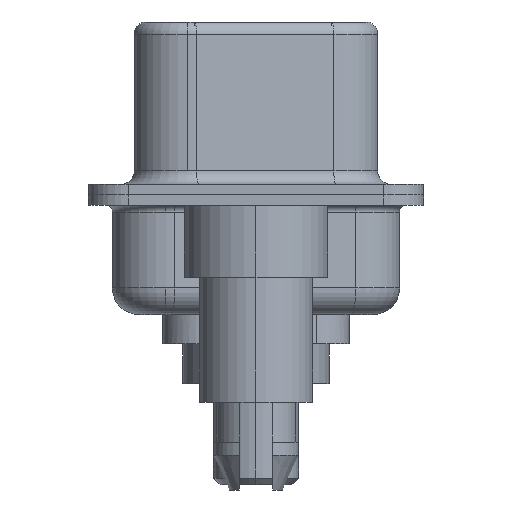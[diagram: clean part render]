
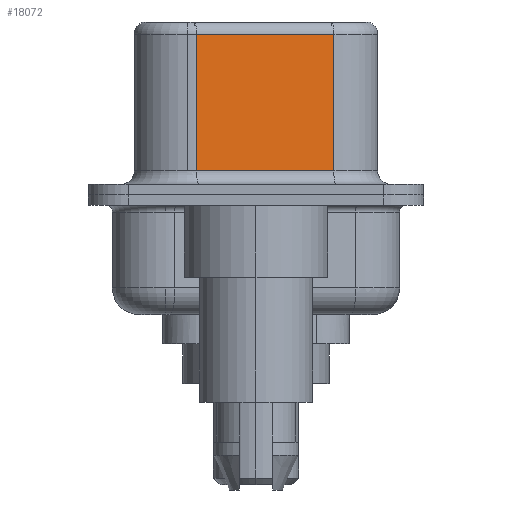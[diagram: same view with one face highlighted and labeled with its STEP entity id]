
A CAD part, left-side view. The second image highlights one B-rep face of the part: STEP entity #18072.
In plain terms, the highlighted planar face has unit normal (-0.985, -0.174, 0).
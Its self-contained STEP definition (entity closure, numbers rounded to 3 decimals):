
#286 = VECTOR ( 'NONE', #8325, 1000. ) ;
#624 = DIRECTION ( 'NONE',  ( 0., 0., -1. ) ) ;
#1634 = LINE ( 'NONE', #17570, #15886 ) ;
#1722 = EDGE_CURVE ( 'NONE', #16612, #19466, #1634, .T. ) ;
#2368 = CARTESIAN_POINT ( 'NONE',  ( 4.58, -2.927, 6.02 ) ) ;
#2498 = CARTESIAN_POINT ( 'NONE',  ( 4.58, -2.927, 0.9 ) ) ;
#3250 = DIRECTION ( 'NONE',  ( 0., 0., -1. ) ) ;
#4191 = VERTEX_POINT ( 'NONE', #2498 ) ;
#4747 = EDGE_CURVE ( 'NONE', #9132, #4191, #20156, .T. ) ;
#6966 = AXIS2_PLACEMENT_3D ( 'NONE', #12024, #13434, #19902 ) ;
#7387 = ORIENTED_EDGE ( 'NONE', *, *, #18178, .F. ) ;
#8325 = DIRECTION ( 'NONE',  ( 0.174, -0.985, 0. ) ) ;
#9132 = VERTEX_POINT ( 'NONE', #19863 ) ;
#9517 = ORIENTED_EDGE ( 'NONE', *, *, #1722, .T. ) ;
#9581 = FACE_OUTER_BOUND ( 'NONE', #17173, .T. ) ;
#10715 = ORIENTED_EDGE ( 'NONE', *, *, #20115, .T. ) ;
#10780 = VECTOR ( 'NONE', #624, 1000. ) ;
#10831 = VECTOR ( 'NONE', #3250, 1000. ) ;
#11376 = CARTESIAN_POINT ( 'NONE',  ( 4.58, -2.927, 6.52 ) ) ;
#12024 = CARTESIAN_POINT ( 'NONE',  ( 4.58, -2.927, 6.52 ) ) ;
#12273 = CARTESIAN_POINT ( 'NONE',  ( 3.67, 2.233, 6.52 ) ) ;
#13434 = DIRECTION ( 'NONE',  ( 0.985, 0.174, 0. ) ) ;
#13480 = CARTESIAN_POINT ( 'NONE',  ( 3.67, 2.233, 6.02 ) ) ;
#15080 = LINE ( 'NONE', #12273, #10780 ) ;
#15687 = LINE ( 'NONE', #11376, #10831 ) ;
#15886 = VECTOR ( 'NONE', #15937, 1000. ) ;
#15937 = DIRECTION ( 'NONE',  ( -0.174, 0.985, 0. ) ) ;
#16178 = ORIENTED_EDGE ( 'NONE', *, *, #4747, .T. ) ;
#16612 = VERTEX_POINT ( 'NONE', #2368 ) ;
#16873 = PLANE ( 'NONE',  #6966 ) ;
#17173 = EDGE_LOOP ( 'NONE', ( #7387, #9517, #10715, #16178 ) ) ;
#17570 = CARTESIAN_POINT ( 'NONE',  ( 4.58, -2.927, 6.02 ) ) ;
#17928 = CARTESIAN_POINT ( 'NONE',  ( 4.58, -2.927, 0.9 ) ) ;
#18072 = ADVANCED_FACE ( 'NONE', ( #9581 ), #16873, .F. ) ;
#18178 = EDGE_CURVE ( 'NONE', #16612, #4191, #15687, .T. ) ;
#19466 = VERTEX_POINT ( 'NONE', #13480 ) ;
#19863 = CARTESIAN_POINT ( 'NONE',  ( 3.67, 2.233, 0.9 ) ) ;
#19902 = DIRECTION ( 'NONE',  ( -0.174, 0.985, 0. ) ) ;
#20115 = EDGE_CURVE ( 'NONE', #19466, #9132, #15080, .T. ) ;
#20156 = LINE ( 'NONE', #17928, #286 ) ;
